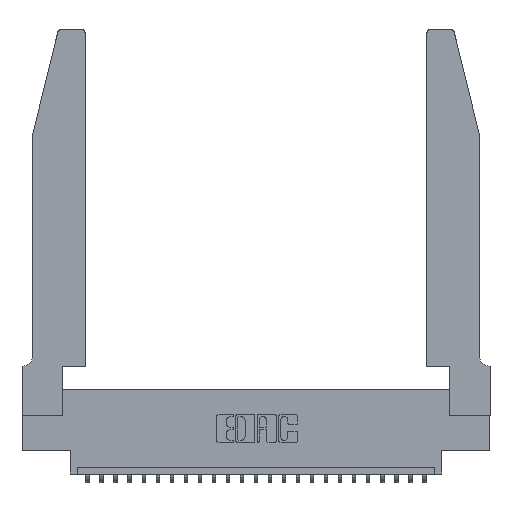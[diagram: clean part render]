
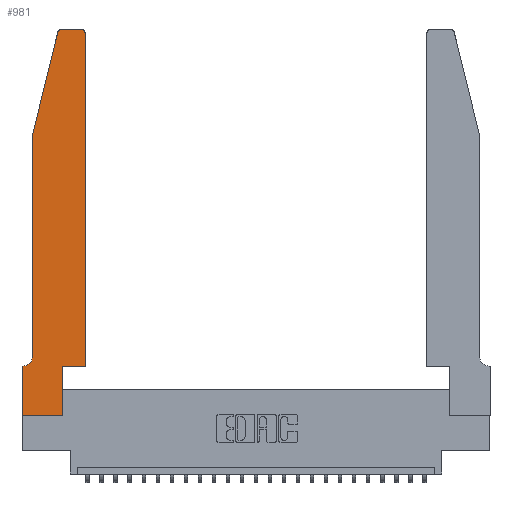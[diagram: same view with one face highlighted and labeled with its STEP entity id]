
A CAD part, top view. The second image highlights one B-rep face of the part: STEP entity #981.
In plain terms, the highlighted planar face has unit normal (0, 0, 1).
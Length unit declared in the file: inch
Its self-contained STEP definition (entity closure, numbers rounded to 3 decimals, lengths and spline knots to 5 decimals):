
#215 = DIRECTION ( 'NONE',  ( 0., 0., 1. ) ) ;
#310 = CARTESIAN_POINT ( 'NONE',  ( 0., 0.35, 0.37 ) ) ;
#439 = EDGE_CURVE ( 'NONE', #5157, #15247, #9695, .T. ) ;
#672 = ORIENTED_EDGE ( 'NONE', *, *, #7760, .T. ) ;
#805 = AXIS2_PLACEMENT_3D ( 'NONE', #22271, #16156, #18169 ) ;
#904 = CARTESIAN_POINT ( 'NONE',  ( 0.4505, 0.35, 0.37 ) ) ;
#981 = ADVANCED_FACE ( 'NONE', ( #19726 ), #18371, .T. ) ;
#988 = CARTESIAN_POINT ( 'NONE',  ( 0.4205, 2.75, 0.37 ) ) ;
#1012 = CARTESIAN_POINT ( 'NONE',  ( 0., 0.35, 0.37 ) ) ;
#1934 = EDGE_CURVE ( 'NONE', #15189, #7610, #13694, .T. ) ;
#2050 = VECTOR ( 'NONE', #4793, 39.37008 ) ;
#2206 = ORIENTED_EDGE ( 'NONE', *, *, #12456, .T. ) ;
#2232 = CARTESIAN_POINT ( 'NONE',  ( 0.4505, 0.35, 0.37 ) ) ;
#2350 = DIRECTION ( 'NONE',  ( 1., 0., 0. ) ) ;
#2745 = ORIENTED_EDGE ( 'NONE', *, *, #10735, .T. ) ;
#2760 = CARTESIAN_POINT ( 'NONE',  ( 0.0055, 0.42, 0.37 ) ) ;
#3030 = ORIENTED_EDGE ( 'NONE', *, *, #6061, .T. ) ;
#3822 = VECTOR ( 'NONE', #12821, 39.37008 ) ;
#3832 = AXIS2_PLACEMENT_3D ( 'NONE', #2760, #6885, #20945 ) ;
#3966 = CARTESIAN_POINT ( 'NONE',  ( 0.2605, 2.75, 0.37 ) ) ;
#4179 = CARTESIAN_POINT ( 'NONE',  ( 0.4505, 2.72, 0.37 ) ) ;
#4209 = LINE ( 'NONE', #16579, #2050 ) ;
#4227 = EDGE_CURVE ( 'NONE', #4790, #23358, #25863, .T. ) ;
#4372 = AXIS2_PLACEMENT_3D ( 'NONE', #14655, #12521, #2350 ) ;
#4570 = CARTESIAN_POINT ( 'NONE',  ( 0.25487, 2.72718, 0.37 ) ) ;
#4790 = VERTEX_POINT ( 'NONE', #4980 ) ;
#4793 = DIRECTION ( 'NONE',  ( 0., -1., 0. ) ) ;
#4974 = LINE ( 'NONE', #3966, #6522 ) ;
#4980 = CARTESIAN_POINT ( 'NONE',  ( 0., 0., 0.37 ) ) ;
#5157 = VERTEX_POINT ( 'NONE', #2232 ) ;
#5906 = CARTESIAN_POINT ( 'NONE',  ( 0.0755, 2., 0.37 ) ) ;
#5949 = LINE ( 'NONE', #904, #20086 ) ;
#6061 = EDGE_CURVE ( 'NONE', #24550, #22663, #23281, .T. ) ;
#6224 = CARTESIAN_POINT ( 'NONE',  ( 0.2865, 0., 0.37 ) ) ;
#6277 = EDGE_CURVE ( 'NONE', #9043, #24550, #22758, .T. ) ;
#6461 = EDGE_CURVE ( 'NONE', #8176, #4790, #9997, .T. ) ;
#6522 = VECTOR ( 'NONE', #8159, 39.37008 ) ;
#6885 = DIRECTION ( 'NONE',  ( 0., 0., -1. ) ) ;
#7399 = DIRECTION ( 'NONE',  ( 0., -1., 0. ) ) ;
#7610 = VERTEX_POINT ( 'NONE', #16140 ) ;
#7760 = EDGE_CURVE ( 'NONE', #15247, #18148, #16884, .T. ) ;
#8159 = DIRECTION ( 'NONE',  ( -1., 0., 0. ) ) ;
#8176 = VERTEX_POINT ( 'NONE', #1012 ) ;
#8318 = DIRECTION ( 'NONE',  ( -1., 0., 0. ) ) ;
#8606 = EDGE_CURVE ( 'NONE', #22663, #15189, #4209, .T. ) ;
#8962 = EDGE_LOOP ( 'NONE', ( #21942, #11147, #3030, #18814, #12287, #14600, #22924, #19282, #2745, #2206, #14325, #672 ) ) ;
#9043 = VERTEX_POINT ( 'NONE', #15692 ) ;
#9165 = DIRECTION ( 'NONE',  ( 1., 0., 0. ) ) ;
#9695 = LINE ( 'NONE', #19647, #20692 ) ;
#9810 = VECTOR ( 'NONE', #25883, 39.37008 ) ;
#9997 = LINE ( 'NONE', #15238, #12497 ) ;
#10735 = EDGE_CURVE ( 'NONE', #23358, #18898, #16392, .T. ) ;
#11147 = ORIENTED_EDGE ( 'NONE', *, *, #6277, .T. ) ;
#11185 = AXIS2_PLACEMENT_3D ( 'NONE', #310, #215, #14404 ) ;
#11571 = EDGE_CURVE ( 'NONE', #7610, #8176, #21711, .T. ) ;
#11964 = CARTESIAN_POINT ( 'NONE',  ( 0.2865, 0.35, 0.37 ) ) ;
#12287 = ORIENTED_EDGE ( 'NONE', *, *, #1934, .T. ) ;
#12456 = EDGE_CURVE ( 'NONE', #18898, #5157, #5949, .T. ) ;
#12497 = VECTOR ( 'NONE', #7399, 39.37008 ) ;
#12521 = DIRECTION ( 'NONE',  ( 0., 0., 1. ) ) ;
#12554 = VECTOR ( 'NONE', #13342, 39.37008 ) ;
#12821 = DIRECTION ( 'NONE',  ( 0., 1., 0. ) ) ;
#13072 = CARTESIAN_POINT ( 'NONE',  ( 0.2865, 0.35, 0.37 ) ) ;
#13342 = DIRECTION ( 'NONE',  ( -0.239, -0.971, 0. ) ) ;
#13694 = CIRCLE ( 'NONE', #3832, 0.07 ) ;
#14325 = ORIENTED_EDGE ( 'NONE', *, *, #439, .T. ) ;
#14404 = DIRECTION ( 'NONE',  ( 1., 0., 0. ) ) ;
#14600 = ORIENTED_EDGE ( 'NONE', *, *, #11571, .T. ) ;
#14655 = CARTESIAN_POINT ( 'NONE',  ( 0.284, 2.72, 0.37 ) ) ;
#15189 = VERTEX_POINT ( 'NONE', #21014 ) ;
#15238 = CARTESIAN_POINT ( 'NONE',  ( 0., 0., 0.37 ) ) ;
#15247 = VERTEX_POINT ( 'NONE', #4179 ) ;
#15692 = CARTESIAN_POINT ( 'NONE',  ( 0.284, 2.75, 0.37 ) ) ;
#16140 = CARTESIAN_POINT ( 'NONE',  ( 0.0055, 0.35, 0.37 ) ) ;
#16156 = DIRECTION ( 'NONE',  ( 0., 0., 1. ) ) ;
#16392 = LINE ( 'NONE', #13072, #3822 ) ;
#16579 = CARTESIAN_POINT ( 'NONE',  ( 0.0755, 2., 0.37 ) ) ;
#16884 = CIRCLE ( 'NONE', #805, 0.03 ) ;
#18148 = VERTEX_POINT ( 'NONE', #988 ) ;
#18169 = DIRECTION ( 'NONE',  ( 1., 0., 0. ) ) ;
#18371 = PLANE ( 'NONE',  #11185 ) ;
#18814 = ORIENTED_EDGE ( 'NONE', *, *, #8606, .T. ) ;
#18884 = VECTOR ( 'NONE', #8318, 39.37008 ) ;
#18898 = VERTEX_POINT ( 'NONE', #11964 ) ;
#19282 = ORIENTED_EDGE ( 'NONE', *, *, #4227, .T. ) ;
#19437 = EDGE_CURVE ( 'NONE', #18148, #9043, #4974, .T. ) ;
#19647 = CARTESIAN_POINT ( 'NONE',  ( 0.4505, 0.35, 0.37 ) ) ;
#19726 = FACE_OUTER_BOUND ( 'NONE', #8962, .T. ) ;
#19739 = DIRECTION ( 'NONE',  ( 0., 1., 0. ) ) ;
#19818 = CARTESIAN_POINT ( 'NONE',  ( 0., 0., 0.37 ) ) ;
#19839 = CARTESIAN_POINT ( 'NONE',  ( 0.0755, 0.35, 0.37 ) ) ;
#20086 = VECTOR ( 'NONE', #9165, 39.37008 ) ;
#20692 = VECTOR ( 'NONE', #19739, 39.37008 ) ;
#20945 = DIRECTION ( 'NONE',  ( -1., 0., 0. ) ) ;
#21014 = CARTESIAN_POINT ( 'NONE',  ( 0.0755, 0.42, 0.37 ) ) ;
#21711 = LINE ( 'NONE', #19839, #18884 ) ;
#21942 = ORIENTED_EDGE ( 'NONE', *, *, #19437, .T. ) ;
#22271 = CARTESIAN_POINT ( 'NONE',  ( 0.4205, 2.72, 0.37 ) ) ;
#22663 = VERTEX_POINT ( 'NONE', #5906 ) ;
#22758 = CIRCLE ( 'NONE', #4372, 0.03 ) ;
#22924 = ORIENTED_EDGE ( 'NONE', *, *, #6461, .T. ) ;
#23281 = LINE ( 'NONE', #25473, #12554 ) ;
#23358 = VERTEX_POINT ( 'NONE', #6224 ) ;
#24550 = VERTEX_POINT ( 'NONE', #4570 ) ;
#25473 = CARTESIAN_POINT ( 'NONE',  ( 0.0755, 2., 0.37 ) ) ;
#25863 = LINE ( 'NONE', #19818, #9810 ) ;
#25883 = DIRECTION ( 'NONE',  ( 1., 0., 0. ) ) ;
